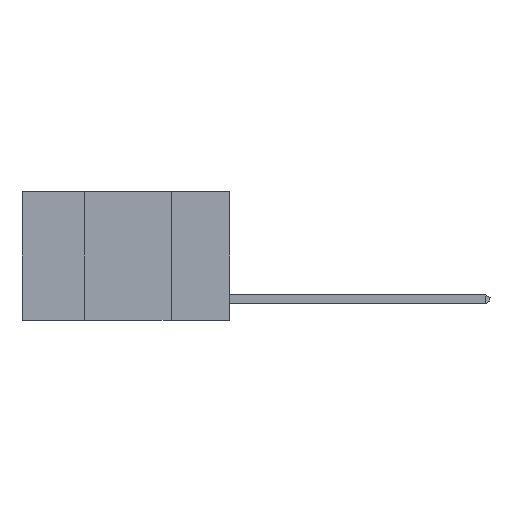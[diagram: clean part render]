
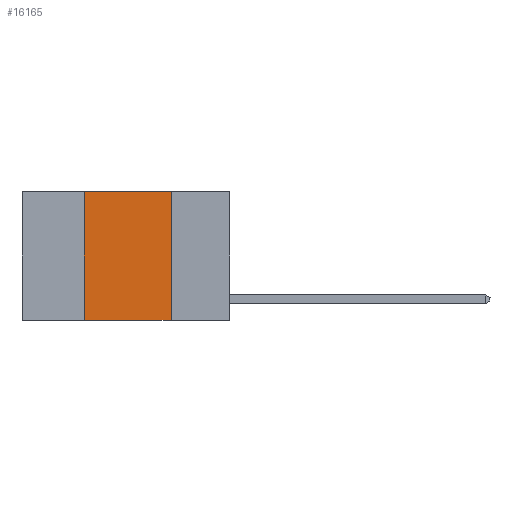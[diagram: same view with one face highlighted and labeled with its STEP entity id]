
A CAD part, left-side view. The second image highlights one B-rep face of the part: STEP entity #16165.
In plain terms, the highlighted planar face has unit normal (-1, 0, 0).
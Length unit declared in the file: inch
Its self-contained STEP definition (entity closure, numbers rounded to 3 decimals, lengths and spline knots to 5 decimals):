
#788 = VECTOR ( 'NONE', #9901, 39.37008 ) ;
#2257 = VERTEX_POINT ( 'NONE', #22984 ) ;
#3372 = CARTESIAN_POINT ( 'NONE',  ( 0., 0.42, 0. ) ) ;
#3549 = EDGE_CURVE ( 'NONE', #5558, #2257, #24151, .T. ) ;
#3972 = PLANE ( 'NONE',  #5713 ) ;
#4300 = VERTEX_POINT ( 'NONE', #8191 ) ;
#4832 = EDGE_CURVE ( 'NONE', #4300, #2257, #6498, .T. ) ;
#5421 = DIRECTION ( 'NONE',  ( 0., 0., 1. ) ) ;
#5558 = VERTEX_POINT ( 'NONE', #11523 ) ;
#5713 = AXIS2_PLACEMENT_3D ( 'NONE', #19658, #11763, #19779 ) ;
#6498 = LINE ( 'NONE', #24436, #18324 ) ;
#6610 = CARTESIAN_POINT ( 'NONE',  ( 0., 0.42, 0. ) ) ;
#6709 = DIRECTION ( 'NONE',  ( 0., -1., 0. ) ) ;
#7146 = EDGE_CURVE ( 'NONE', #5558, #22119, #7196, .T. ) ;
#7196 = LINE ( 'NONE', #3372, #17669 ) ;
#8191 = CARTESIAN_POINT ( 'NONE',  ( 0., 0.17, 0. ) ) ;
#9777 = LINE ( 'NONE', #15513, #788 ) ;
#9901 = DIRECTION ( 'NONE',  ( 0., -1., 0. ) ) ;
#11523 = CARTESIAN_POINT ( 'NONE',  ( 0., 0.42, -0.37 ) ) ;
#11763 = DIRECTION ( 'NONE',  ( 1., 0., 0. ) ) ;
#12525 = ORIENTED_EDGE ( 'NONE', *, *, #22450, .F. ) ;
#13764 = ORIENTED_EDGE ( 'NONE', *, *, #4832, .F. ) ;
#15513 = CARTESIAN_POINT ( 'NONE',  ( 0., 0.6, 0. ) ) ;
#16154 = ORIENTED_EDGE ( 'NONE', *, *, #3549, .T. ) ;
#16165 = ADVANCED_FACE ( 'NONE', ( #21938 ), #3972, .F. ) ;
#16764 = CARTESIAN_POINT ( 'NONE',  ( 0., 0.6, -0.37 ) ) ;
#17669 = VECTOR ( 'NONE', #5421, 39.37008 ) ;
#18324 = VECTOR ( 'NONE', #22278, 39.37008 ) ;
#19658 = CARTESIAN_POINT ( 'NONE',  ( 0., 0.6, 0. ) ) ;
#19779 = DIRECTION ( 'NONE',  ( 0., 0., -1. ) ) ;
#19814 = EDGE_LOOP ( 'NONE', ( #13764, #12525, #24239, #16154 ) ) ;
#21083 = VECTOR ( 'NONE', #6709, 39.37008 ) ;
#21938 = FACE_OUTER_BOUND ( 'NONE', #19814, .T. ) ;
#22119 = VERTEX_POINT ( 'NONE', #6610 ) ;
#22278 = DIRECTION ( 'NONE',  ( 0., 0., -1. ) ) ;
#22450 = EDGE_CURVE ( 'NONE', #22119, #4300, #9777, .T. ) ;
#22984 = CARTESIAN_POINT ( 'NONE',  ( 0., 0.17, -0.37 ) ) ;
#24151 = LINE ( 'NONE', #16764, #21083 ) ;
#24239 = ORIENTED_EDGE ( 'NONE', *, *, #7146, .F. ) ;
#24436 = CARTESIAN_POINT ( 'NONE',  ( 0., 0.17, 0. ) ) ;
